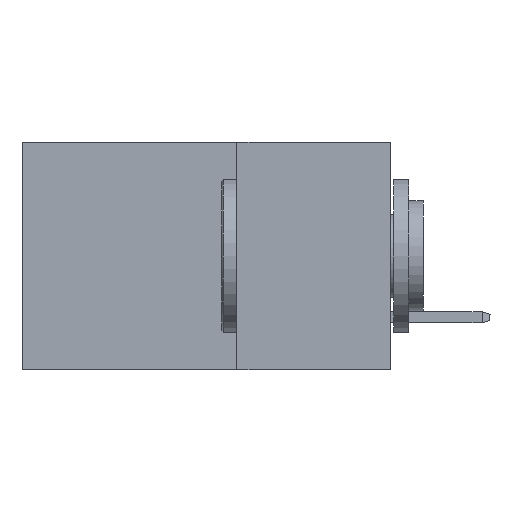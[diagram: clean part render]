
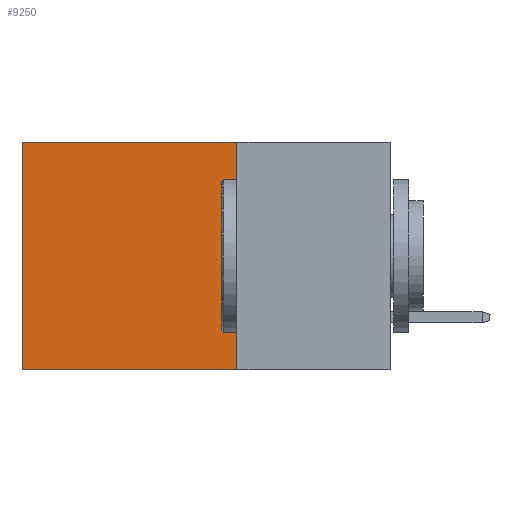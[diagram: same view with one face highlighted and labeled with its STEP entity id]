
A CAD part, left-side view. The second image highlights one B-rep face of the part: STEP entity #9250.
In plain terms, the highlighted planar face has unit normal (-1, 0, 0).
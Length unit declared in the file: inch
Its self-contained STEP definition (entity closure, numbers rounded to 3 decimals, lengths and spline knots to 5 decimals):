
#16 = CARTESIAN_POINT ( 'NONE',  ( 0.2875, 0.25, 0. ) ) ;
#40 = VECTOR ( 'NONE', #16109, 39.37008 ) ;
#756 = EDGE_CURVE ( 'NONE', #6385, #13072, #18459, .T. ) ;
#2885 = CARTESIAN_POINT ( 'NONE',  ( 0.2875, 0.25, -0.37 ) ) ;
#4059 = EDGE_CURVE ( 'NONE', #13072, #10118, #17331, .T. ) ;
#4371 = DIRECTION ( 'NONE',  ( 0., 0., -1. ) ) ;
#5686 = CARTESIAN_POINT ( 'NONE',  ( 0.2875, 0.25, 0. ) ) ;
#6087 = CARTESIAN_POINT ( 'NONE',  ( 0.2875, 0.25, 0. ) ) ;
#6236 = ORIENTED_EDGE ( 'NONE', *, *, #4059, .T. ) ;
#6385 = VERTEX_POINT ( 'NONE', #6087 ) ;
#6597 = ORIENTED_EDGE ( 'NONE', *, *, #756, .T. ) ;
#7457 = VECTOR ( 'NONE', #19532, 39.37008 ) ;
#8193 = CARTESIAN_POINT ( 'NONE',  ( 0.2875, 0.25, -0.37 ) ) ;
#8204 = EDGE_CURVE ( 'NONE', #6385, #13208, #23031, .T. ) ;
#8772 = CARTESIAN_POINT ( 'NONE',  ( 0.2875, 0.6, 0. ) ) ;
#9250 = ADVANCED_FACE ( 'NONE', ( #17655 ), #11875, .F. ) ;
#10118 = VERTEX_POINT ( 'NONE', #14108 ) ;
#11079 = EDGE_CURVE ( 'NONE', #13208, #10118, #11777, .T. ) ;
#11754 = VECTOR ( 'NONE', #4371, 39.37008 ) ;
#11777 = LINE ( 'NONE', #2885, #40 ) ;
#11798 = DIRECTION ( 'NONE',  ( 0., 0., -1. ) ) ;
#11875 = PLANE ( 'NONE',  #12044 ) ;
#11984 = EDGE_LOOP ( 'NONE', ( #6236, #20900, #20912, #6597 ) ) ;
#12044 = AXIS2_PLACEMENT_3D ( 'NONE', #21167, #23053, #11798 ) ;
#13072 = VERTEX_POINT ( 'NONE', #16016 ) ;
#13208 = VERTEX_POINT ( 'NONE', #8193 ) ;
#13459 = VECTOR ( 'NONE', #15097, 39.37008 ) ;
#14108 = CARTESIAN_POINT ( 'NONE',  ( 0.2875, 0.6, -0.37 ) ) ;
#15097 = DIRECTION ( 'NONE',  ( 0., 1., 0. ) ) ;
#16016 = CARTESIAN_POINT ( 'NONE',  ( 0.2875, 0.6, 0. ) ) ;
#16109 = DIRECTION ( 'NONE',  ( 0., 1., 0. ) ) ;
#17331 = LINE ( 'NONE', #8772, #11754 ) ;
#17655 = FACE_OUTER_BOUND ( 'NONE', #11984, .T. ) ;
#18459 = LINE ( 'NONE', #16, #13459 ) ;
#19532 = DIRECTION ( 'NONE',  ( 0., 0., -1. ) ) ;
#20900 = ORIENTED_EDGE ( 'NONE', *, *, #11079, .F. ) ;
#20912 = ORIENTED_EDGE ( 'NONE', *, *, #8204, .F. ) ;
#21167 = CARTESIAN_POINT ( 'NONE',  ( 0.2875, 0.25, 0. ) ) ;
#23031 = LINE ( 'NONE', #5686, #7457 ) ;
#23053 = DIRECTION ( 'NONE',  ( 1., 0., 0. ) ) ;
